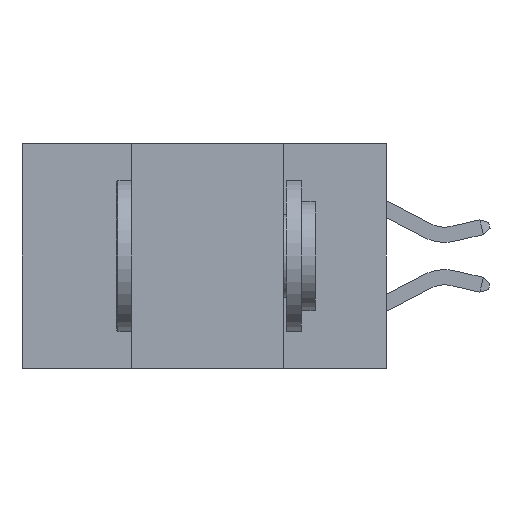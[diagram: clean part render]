
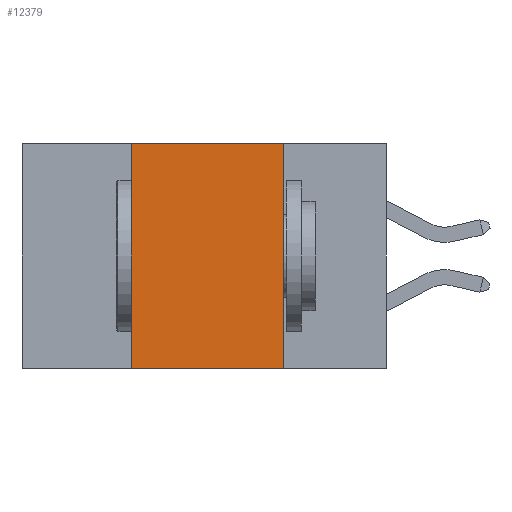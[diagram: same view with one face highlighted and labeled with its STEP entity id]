
A CAD part, left-side view. The second image highlights one B-rep face of the part: STEP entity #12379.
In plain terms, the highlighted planar face has unit normal (-1, 0, 0).
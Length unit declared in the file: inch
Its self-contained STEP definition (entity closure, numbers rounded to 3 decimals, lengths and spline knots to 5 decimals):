
#63 = CARTESIAN_POINT ( 'NONE',  ( 0., 0.17, -0.37 ) ) ;
#803 = VECTOR ( 'NONE', #16921, 39.37008 ) ;
#1740 = CARTESIAN_POINT ( 'NONE',  ( 0., 0.42, -0.37 ) ) ;
#1869 = EDGE_LOOP ( 'NONE', ( #21119, #20388, #16337, #2493 ) ) ;
#2493 = ORIENTED_EDGE ( 'NONE', *, *, #18095, .T. ) ;
#3190 = LINE ( 'NONE', #16819, #803 ) ;
#3856 = VECTOR ( 'NONE', #19192, 39.37008 ) ;
#4106 = EDGE_CURVE ( 'NONE', #11508, #21037, #3190, .T. ) ;
#4794 = EDGE_CURVE ( 'NONE', #21037, #19157, #19118, .T. ) ;
#4829 = PLANE ( 'NONE',  #16690 ) ;
#5375 = CARTESIAN_POINT ( 'NONE',  ( 0., 0.17, -0.37 ) ) ;
#5891 = CARTESIAN_POINT ( 'NONE',  ( 0., 0.42, -0.37 ) ) ;
#6271 = DIRECTION ( 'NONE',  ( 1., 0., 0. ) ) ;
#6444 = CARTESIAN_POINT ( 'NONE',  ( 0., 0.17, 0. ) ) ;
#10688 = DIRECTION ( 'NONE',  ( 0., 0., -1. ) ) ;
#11369 = DIRECTION ( 'NONE',  ( 0., 0., -1. ) ) ;
#11508 = VERTEX_POINT ( 'NONE', #21125 ) ;
#12379 = ADVANCED_FACE ( 'NONE', ( #18008 ), #4829, .F. ) ;
#12534 = LINE ( 'NONE', #5891, #3856 ) ;
#13130 = EDGE_CURVE ( 'NONE', #14843, #11508, #12534, .T. ) ;
#13274 = VECTOR ( 'NONE', #10688, 39.37008 ) ;
#13674 = DIRECTION ( 'NONE',  ( 0., -1., 0. ) ) ;
#14843 = VERTEX_POINT ( 'NONE', #1740 ) ;
#16337 = ORIENTED_EDGE ( 'NONE', *, *, #13130, .F. ) ;
#16690 = AXIS2_PLACEMENT_3D ( 'NONE', #18238, #6271, #11369 ) ;
#16819 = CARTESIAN_POINT ( 'NONE',  ( 0., 0.6, 0. ) ) ;
#16921 = DIRECTION ( 'NONE',  ( 0., -1., 0. ) ) ;
#16987 = CARTESIAN_POINT ( 'NONE',  ( 0., 0.6, -0.37 ) ) ;
#18008 = FACE_OUTER_BOUND ( 'NONE', #1869, .T. ) ;
#18095 = EDGE_CURVE ( 'NONE', #14843, #19157, #18657, .T. ) ;
#18238 = CARTESIAN_POINT ( 'NONE',  ( 0., 0.6, 0. ) ) ;
#18622 = VECTOR ( 'NONE', #13674, 39.37008 ) ;
#18657 = LINE ( 'NONE', #16987, #18622 ) ;
#19118 = LINE ( 'NONE', #5375, #13274 ) ;
#19157 = VERTEX_POINT ( 'NONE', #63 ) ;
#19192 = DIRECTION ( 'NONE',  ( 0., 0., 1. ) ) ;
#20388 = ORIENTED_EDGE ( 'NONE', *, *, #4106, .F. ) ;
#21037 = VERTEX_POINT ( 'NONE', #6444 ) ;
#21119 = ORIENTED_EDGE ( 'NONE', *, *, #4794, .F. ) ;
#21125 = CARTESIAN_POINT ( 'NONE',  ( 0., 0.42, 0. ) ) ;
